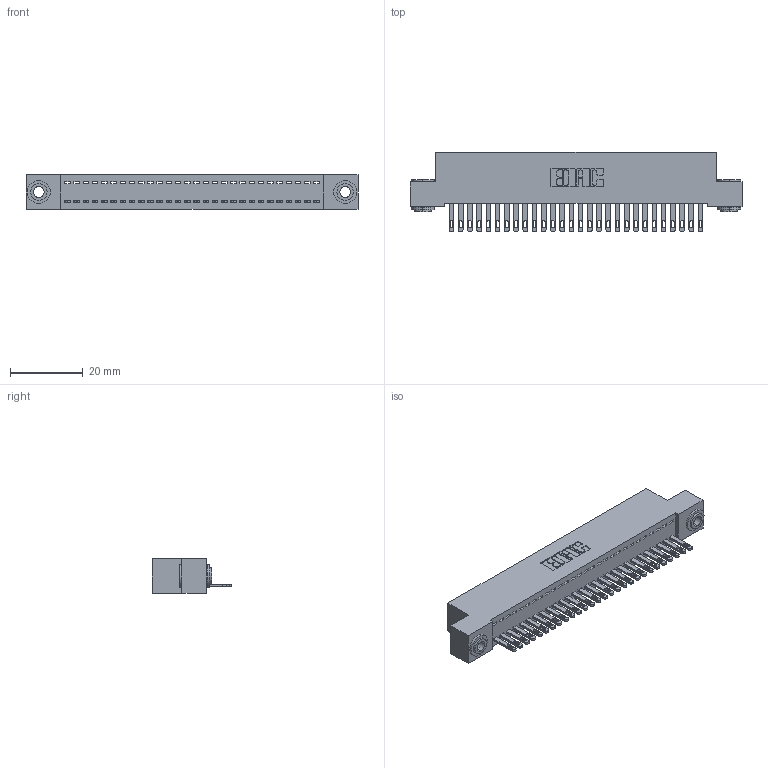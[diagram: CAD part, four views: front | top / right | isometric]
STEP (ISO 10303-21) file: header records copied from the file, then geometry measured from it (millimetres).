
FILE_DESCRIPTION (( 'STEP AP203' ), '1' );
FILE_NAME ('342-028-500-103.STEP', '2018-08-11T06:04:58', ( '' ), ( '' ), 'SwSTEP 2.0', 'SolidWorks 2016', '' );
FILE_SCHEMA (( 'CONFIG_CONTROL_DESIGN' ));
Length unit declared in the file: inch
Products named in the file (4): 342 Part_.156 TH; 345-292-001_345-293-100; 342-250-002_345-250-002-102; 342-028-500-103
Assembly tree (31 placements, depth 2):
  342-028-500-103
    342 Part_.156 TH
    345-292-001_345-293-100  x28
    342-250-002_345-250-002-102  x2
Bounding box: 91.44 x 21.85 x 9.4 mm (x, y, z)
Volume: 8006 mm3; surface area: 11776.4 mm2
Topology: 31 solids, 31 shells, 1660 faces, 5079 edges, 3382 vertices
Faces by surface type: plane 1084, cylinder 568, cone 8
Entity records: 19376 total; most frequent: CARTESIAN_POINT 3321, ORIENTED_EDGE 3278, DIRECTION 2865, EDGE_CURVE 1639, LINE 1483, VECTOR 1483, VERTEX_POINT 1090, AXIS2_PLACEMENT_3D 691
